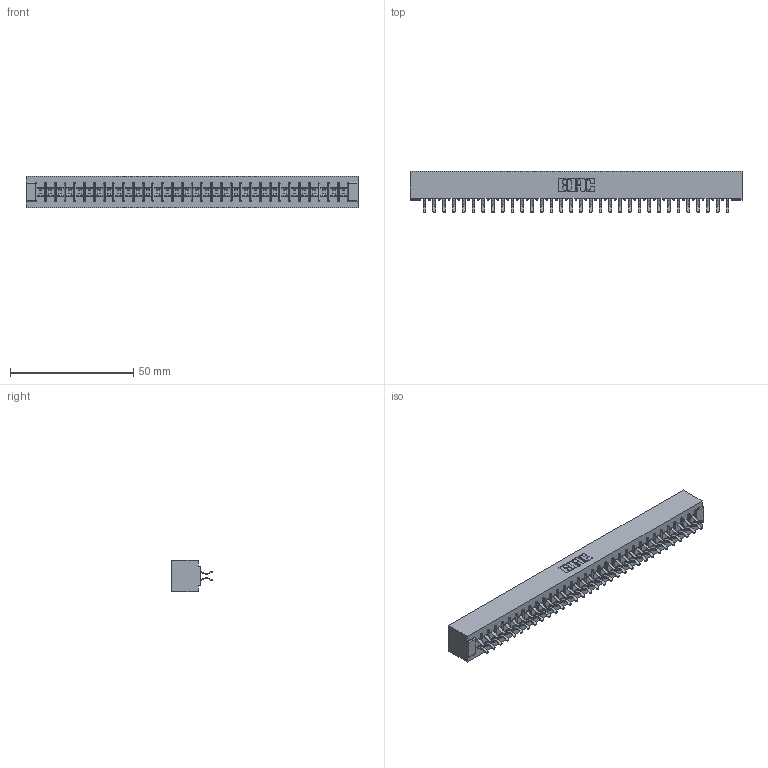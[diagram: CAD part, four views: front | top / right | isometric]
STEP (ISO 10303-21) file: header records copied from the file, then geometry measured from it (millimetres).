
FILE_DESCRIPTION (( 'STEP AP203' ), '1' );
FILE_NAME ('315-064-556-201.STEP', '2019-09-10T20:39:37', ( '' ), ( '' ), 'SwSTEP 2.0', 'SolidWorks 2016', '' );
FILE_SCHEMA (( 'CONFIG_CONTROL_DESIGN' ));
Length unit declared in the file: inch
Products named in the file (3): 315-064-556-201; 305-290-001_556; 305 Part_No Mounting
Assembly tree (65 placements, depth 2):
  315-064-556-201
    305 Part_No Mounting
    305-290-001_556  x64
Bounding box: 134.67 x 16.64 x 12.7 mm (x, y, z)
Volume: 14467.8 mm3; surface area: 18596.2 mm2
Topology: 65 solids, 65 shells, 3692 faces, 10628 edges, 6912 vertices
Faces by surface type: plane 2048, cylinder 1516, sphere 128
Entity records: 35809 total; most frequent: CARTESIAN_POINT 5926, ORIENTED_EDGE 5880, DIRECTION 5742, EDGE_CURVE 2940, VECTOR 2366, LINE 2366, VERTEX_POINT 1872, AXIS2_PLACEMENT_3D 1688
